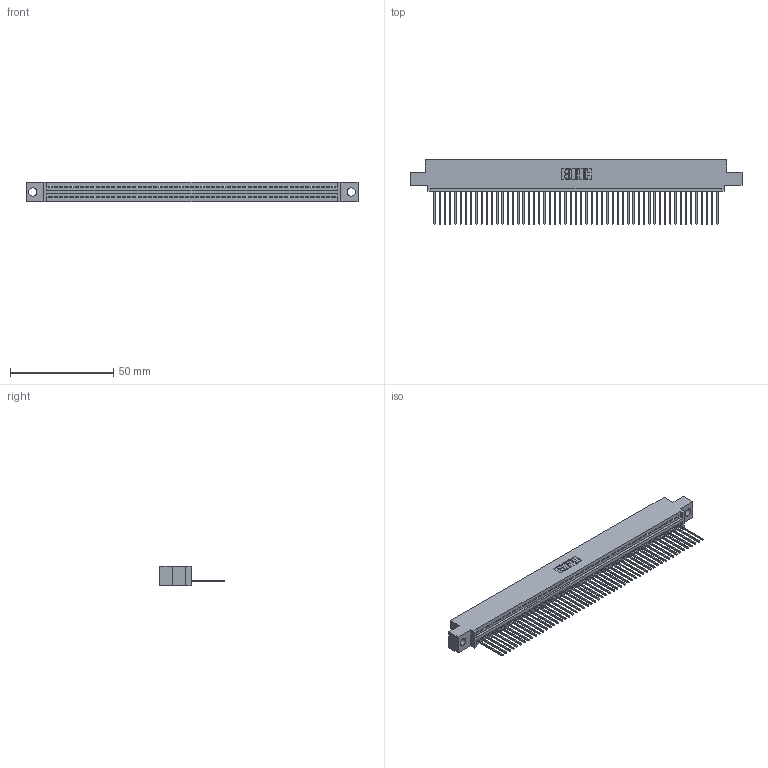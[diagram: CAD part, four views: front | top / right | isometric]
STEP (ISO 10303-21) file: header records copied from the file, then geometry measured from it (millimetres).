
FILE_DESCRIPTION (( 'STEP AP203' ), '1' );
FILE_NAME ('395-055-542-404.STEP', '2021-05-31T21:36:21', ( '' ), ( '' ), 'SwSTEP 2.0', 'SolidWorks 2020', '' );
FILE_SCHEMA (( 'CONFIG_CONTROL_DESIGN' ));
Length unit declared in the file: inch
Products named in the file (3): 395-055-542-404; 345 Part_0.110 Offset - 0.156 Dia-TI; 345-292-001_345-293-142
Assembly tree (56 placements, depth 2):
  395-055-542-404
    345 Part_0.110 Offset - 0.156 Dia-TI
    345-292-001_345-293-142  x55
Bounding box: 160.91 x 31.29 x 9.4 mm (x, y, z)
Volume: 15332.8 mm3; surface area: 21250.9 mm2
Topology: 56 solids, 56 shells, 3334 faces, 10069 edges, 6638 vertices
Faces by surface type: plane 2298, cylinder 1036
Entity records: 40213 total; most frequent: CARTESIAN_POINT 6975, ORIENTED_EDGE 6962, DIRECTION 6071, EDGE_CURVE 3481, VECTOR 3129, LINE 3129, VERTEX_POINT 2318, AXIS2_PLACEMENT_3D 1471
